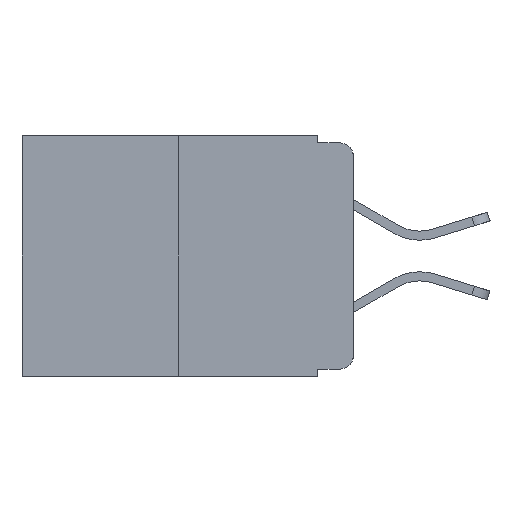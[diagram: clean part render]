
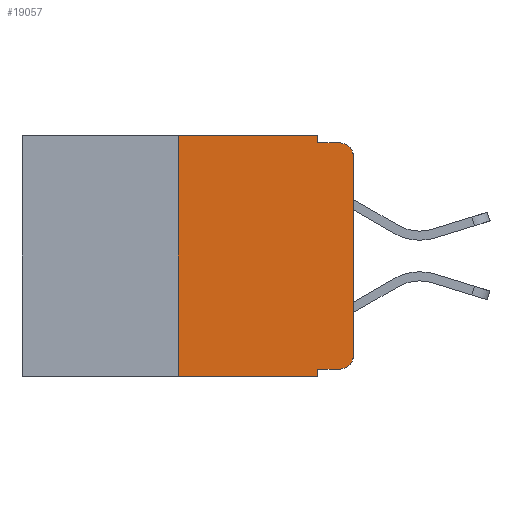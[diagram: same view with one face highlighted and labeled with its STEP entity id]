
A CAD part, left-side view. The second image highlights one B-rep face of the part: STEP entity #19057.
In plain terms, the highlighted planar face has unit normal (-1, 0, 0).
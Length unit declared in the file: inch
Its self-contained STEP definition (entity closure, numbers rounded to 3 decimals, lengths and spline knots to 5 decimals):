
#191 = DIRECTION ( 'NONE',  ( 0., -1., 0. ) ) ;
#465 = DIRECTION ( 'NONE',  ( 0., -1., 0. ) ) ;
#713 = CARTESIAN_POINT ( 'NONE',  ( 0., 0.25, 0. ) ) ;
#757 = VECTOR ( 'NONE', #18524, 39.37008 ) ;
#1115 = AXIS2_PLACEMENT_3D ( 'NONE', #14536, #14515, #14653 ) ;
#1253 = CARTESIAN_POINT ( 'NONE',  ( 0., 0.051, 0. ) ) ;
#1798 = DIRECTION ( 'NONE',  ( 0., 0., -1. ) ) ;
#1947 = CARTESIAN_POINT ( 'NONE',  ( 0., 0.473, 0. ) ) ;
#2078 = CARTESIAN_POINT ( 'NONE',  ( 0., 0., -0.03 ) ) ;
#2240 = CARTESIAN_POINT ( 'NONE',  ( 0., 0.051, -0.01 ) ) ;
#2393 = ORIENTED_EDGE ( 'NONE', *, *, #8087, .T. ) ;
#2534 = VERTEX_POINT ( 'NONE', #5169 ) ;
#2618 = DIRECTION ( 'NONE',  ( 0., 0., 1. ) ) ;
#3215 = CARTESIAN_POINT ( 'NONE',  ( 0., 0.051, -0.343 ) ) ;
#3396 = VECTOR ( 'NONE', #14145, 39.37008 ) ;
#3618 = LINE ( 'NONE', #15783, #7481 ) ;
#3978 = EDGE_LOOP ( 'NONE', ( #6505, #7108, #21864, #22426, #8881, #19845, #6208, #11258, #2393, #8005 ) ) ;
#4554 = DIRECTION ( 'NONE',  ( 0., 0., -1. ) ) ;
#4785 = VERTEX_POINT ( 'NONE', #12264 ) ;
#5070 = EDGE_CURVE ( 'NONE', #6015, #2534, #21597, .T. ) ;
#5169 = CARTESIAN_POINT ( 'NONE',  ( 0., 0.02, -0.01 ) ) ;
#5239 = CARTESIAN_POINT ( 'NONE',  ( 0., 0.051, 0. ) ) ;
#5549 = EDGE_CURVE ( 'NONE', #14625, #23654, #16715, .T. ) ;
#5665 = CARTESIAN_POINT ( 'NONE',  ( 0., 0.473, 0. ) ) ;
#5750 = PLANE ( 'NONE',  #12370 ) ;
#6015 = VERTEX_POINT ( 'NONE', #2078 ) ;
#6208 = ORIENTED_EDGE ( 'NONE', *, *, #16862, .T. ) ;
#6269 = CARTESIAN_POINT ( 'NONE',  ( 0., 0.25, -0.343 ) ) ;
#6505 = ORIENTED_EDGE ( 'NONE', *, *, #23655, .T. ) ;
#6599 = CARTESIAN_POINT ( 'NONE',  ( 0., 0.473, -0.343 ) ) ;
#6793 = VECTOR ( 'NONE', #1798, 39.37008 ) ;
#7108 = ORIENTED_EDGE ( 'NONE', *, *, #5070, .T. ) ;
#7127 = DIRECTION ( 'NONE',  ( -1., 0., 0. ) ) ;
#7481 = VECTOR ( 'NONE', #4554, 39.37008 ) ;
#7674 = DIRECTION ( 'NONE',  ( 1., 0., 0. ) ) ;
#7934 = DIRECTION ( 'NONE',  ( 0., 0., 1. ) ) ;
#8005 = ORIENTED_EDGE ( 'NONE', *, *, #9247, .T. ) ;
#8087 = EDGE_CURVE ( 'NONE', #23172, #8336, #16893, .T. ) ;
#8336 = VERTEX_POINT ( 'NONE', #19218 ) ;
#8881 = ORIENTED_EDGE ( 'NONE', *, *, #14238, .F. ) ;
#9183 = VECTOR ( 'NONE', #2618, 39.37008 ) ;
#9247 = EDGE_CURVE ( 'NONE', #8336, #17991, #15163, .T. ) ;
#9855 = VERTEX_POINT ( 'NONE', #3215 ) ;
#10160 = VECTOR ( 'NONE', #7934, 39.37008 ) ;
#11258 = ORIENTED_EDGE ( 'NONE', *, *, #18018, .F. ) ;
#12264 = CARTESIAN_POINT ( 'NONE',  ( 0., 0.25, 0. ) ) ;
#12370 = AXIS2_PLACEMENT_3D ( 'NONE', #5665, #7674, #20590 ) ;
#13857 = CARTESIAN_POINT ( 'NONE',  ( 0., 0., -0.313 ) ) ;
#13924 = CARTESIAN_POINT ( 'NONE',  ( 0., 0.051, -0.333 ) ) ;
#14145 = DIRECTION ( 'NONE',  ( 0., -1., 0. ) ) ;
#14238 = EDGE_CURVE ( 'NONE', #4785, #14625, #19101, .T. ) ;
#14455 = FACE_OUTER_BOUND ( 'NONE', #3978, .T. ) ;
#14515 = DIRECTION ( 'NONE',  ( -1., 0., 0. ) ) ;
#14536 = CARTESIAN_POINT ( 'NONE',  ( 0., 0.02, -0.03 ) ) ;
#14573 = LINE ( 'NONE', #6599, #3396 ) ;
#14625 = VERTEX_POINT ( 'NONE', #1253 ) ;
#14653 = DIRECTION ( 'NONE',  ( 0., 0., -1. ) ) ;
#14888 = CARTESIAN_POINT ( 'NONE',  ( 0., 0.051, -0.333 ) ) ;
#15114 = LINE ( 'NONE', #15366, #10160 ) ;
#15163 = CIRCLE ( 'NONE', #22610, 0.02 ) ;
#15366 = CARTESIAN_POINT ( 'NONE',  ( 0., 0., 0. ) ) ;
#15428 = CARTESIAN_POINT ( 'NONE',  ( 0., 0.051, -0.01 ) ) ;
#15783 = CARTESIAN_POINT ( 'NONE',  ( 0., 0.051, 0. ) ) ;
#16715 = LINE ( 'NONE', #5239, #6793 ) ;
#16751 = VERTEX_POINT ( 'NONE', #6269 ) ;
#16862 = EDGE_CURVE ( 'NONE', #16751, #9855, #14573, .T. ) ;
#16893 = LINE ( 'NONE', #14888, #757 ) ;
#17991 = VERTEX_POINT ( 'NONE', #13857 ) ;
#18018 = EDGE_CURVE ( 'NONE', #23172, #9855, #3618, .T. ) ;
#18234 = CARTESIAN_POINT ( 'NONE',  ( 0., 0.02, -0.313 ) ) ;
#18524 = DIRECTION ( 'NONE',  ( 0., -1., 0. ) ) ;
#18532 = VECTOR ( 'NONE', #191, 39.37008 ) ;
#19057 = ADVANCED_FACE ( 'NONE', ( #14455 ), #5750, .F. ) ;
#19101 = LINE ( 'NONE', #1947, #18532 ) ;
#19218 = CARTESIAN_POINT ( 'NONE',  ( 0., 0.02, -0.333 ) ) ;
#19235 = EDGE_CURVE ( 'NONE', #16751, #4785, #23810, .T. ) ;
#19845 = ORIENTED_EDGE ( 'NONE', *, *, #19235, .F. ) ;
#20065 = DIRECTION ( 'NONE',  ( 0., 0., -1. ) ) ;
#20590 = DIRECTION ( 'NONE',  ( 0., 0., -1. ) ) ;
#20922 = EDGE_CURVE ( 'NONE', #23654, #2534, #23217, .T. ) ;
#21597 = CIRCLE ( 'NONE', #1115, 0.02 ) ;
#21864 = ORIENTED_EDGE ( 'NONE', *, *, #20922, .F. ) ;
#22426 = ORIENTED_EDGE ( 'NONE', *, *, #5549, .F. ) ;
#22610 = AXIS2_PLACEMENT_3D ( 'NONE', #18234, #7127, #20065 ) ;
#22662 = VECTOR ( 'NONE', #465, 39.37008 ) ;
#23172 = VERTEX_POINT ( 'NONE', #13924 ) ;
#23217 = LINE ( 'NONE', #15428, #22662 ) ;
#23654 = VERTEX_POINT ( 'NONE', #2240 ) ;
#23655 = EDGE_CURVE ( 'NONE', #17991, #6015, #15114, .T. ) ;
#23810 = LINE ( 'NONE', #713, #9183 ) ;
